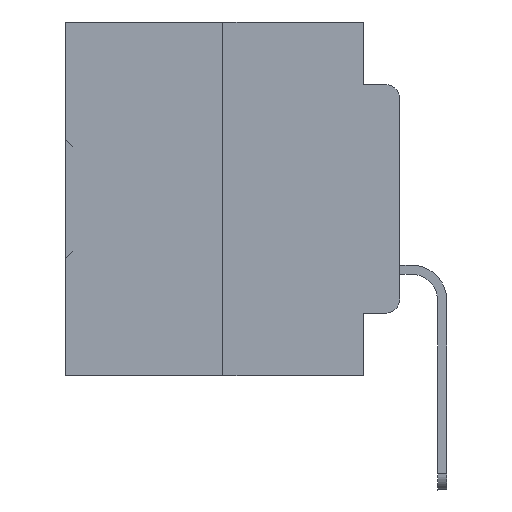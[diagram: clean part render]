
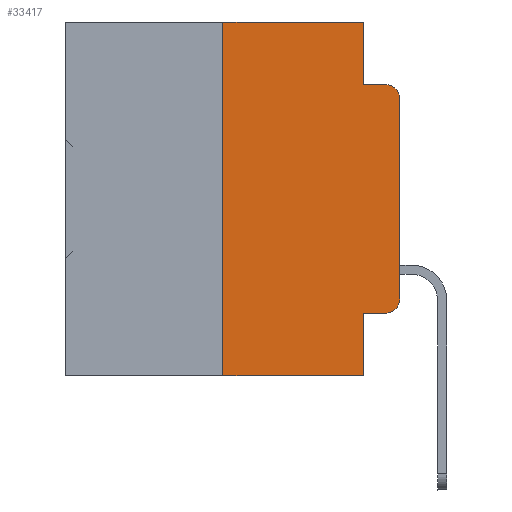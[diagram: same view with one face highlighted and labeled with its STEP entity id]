
A CAD part, left-side view. The second image highlights one B-rep face of the part: STEP entity #33417.
In plain terms, the highlighted planar face has unit normal (-1, 0, 0).
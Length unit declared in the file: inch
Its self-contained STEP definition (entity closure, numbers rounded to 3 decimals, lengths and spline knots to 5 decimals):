
#557 = EDGE_CURVE ( 'NONE', #13613, #4150, #12148, .T. ) ;
#837 = DIRECTION ( 'NONE',  ( 0., -1., 0. ) ) ;
#1370 = VERTEX_POINT ( 'NONE', #20923 ) ;
#1842 = AXIS2_PLACEMENT_3D ( 'NONE', #28471, #22711, #34434 ) ;
#2029 = CARTESIAN_POINT ( 'NONE',  ( 0., 0.02, -0.0885 ) ) ;
#2044 = FACE_OUTER_BOUND ( 'NONE', #7309, .T. ) ;
#2407 = DIRECTION ( 'NONE',  ( -1., 0., 0. ) ) ;
#2476 = ORIENTED_EDGE ( 'NONE', *, *, #37517, .F. ) ;
#2624 = DIRECTION ( 'NONE',  ( 1., 0., 0. ) ) ;
#3008 = EDGE_CURVE ( 'NONE', #10098, #31076, #10506, .T. ) ;
#3671 = EDGE_CURVE ( 'NONE', #20404, #1370, #37446, .T. ) ;
#4150 = VERTEX_POINT ( 'NONE', #14143 ) ;
#4730 = LINE ( 'NONE', #36672, #31308 ) ;
#4738 = CARTESIAN_POINT ( 'NONE',  ( 0., 0.473, 0. ) ) ;
#4822 = ORIENTED_EDGE ( 'NONE', *, *, #557, .F. ) ;
#4982 = AXIS2_PLACEMENT_3D ( 'NONE', #4738, #2624, #28810 ) ;
#5574 = CARTESIAN_POINT ( 'NONE',  ( 0., 0.051, -0.0885 ) ) ;
#5690 = ORIENTED_EDGE ( 'NONE', *, *, #16403, .F. ) ;
#6623 = LINE ( 'NONE', #18384, #8568 ) ;
#7309 = EDGE_LOOP ( 'NONE', ( #28103, #14606, #2476, #34614, #4822, #5690, #7609, #26396, #16035, #16125 ) ) ;
#7523 = VECTOR ( 'NONE', #33469, 39.37008 ) ;
#7609 = ORIENTED_EDGE ( 'NONE', *, *, #3671, .T. ) ;
#7695 = CARTESIAN_POINT ( 'NONE',  ( 0., 0.25, -0.5 ) ) ;
#8011 = DIRECTION ( 'NONE',  ( 0., 0., 1. ) ) ;
#8186 = CARTESIAN_POINT ( 'NONE',  ( 0., 0.02, -0.4115 ) ) ;
#8386 = VERTEX_POINT ( 'NONE', #29024 ) ;
#8568 = VECTOR ( 'NONE', #837, 39.37008 ) ;
#8943 = CARTESIAN_POINT ( 'NONE',  ( 0., 0., -0.3915 ) ) ;
#9642 = VECTOR ( 'NONE', #28596, 39.37008 ) ;
#10098 = VERTEX_POINT ( 'NONE', #8186 ) ;
#10496 = EDGE_CURVE ( 'NONE', #18296, #1370, #11603, .T. ) ;
#10506 = CIRCLE ( 'NONE', #24674, 0.02 ) ;
#11361 = VERTEX_POINT ( 'NONE', #5574 ) ;
#11523 = DIRECTION ( 'NONE',  ( 0., 0., -1. ) ) ;
#11603 = LINE ( 'NONE', #20277, #32957 ) ;
#12123 = VECTOR ( 'NONE', #11523, 39.37008 ) ;
#12148 = LINE ( 'NONE', #23902, #27666 ) ;
#13613 = VERTEX_POINT ( 'NONE', #27407 ) ;
#14143 = CARTESIAN_POINT ( 'NONE',  ( 0., 0.051, 0. ) ) ;
#14606 = ORIENTED_EDGE ( 'NONE', *, *, #38030, .T. ) ;
#16035 = ORIENTED_EDGE ( 'NONE', *, *, #32227, .T. ) ;
#16125 = ORIENTED_EDGE ( 'NONE', *, *, #3008, .T. ) ;
#16403 = EDGE_CURVE ( 'NONE', #20404, #13613, #16863, .T. ) ;
#16815 = DIRECTION ( 'NONE',  ( 0., 0., -1. ) ) ;
#16863 = LINE ( 'NONE', #34179, #9642 ) ;
#18296 = VERTEX_POINT ( 'NONE', #21407 ) ;
#18384 = CARTESIAN_POINT ( 'NONE',  ( 0., 0.051, -0.0885 ) ) ;
#19117 = EDGE_CURVE ( 'NONE', #4150, #11361, #19825, .T. ) ;
#19825 = LINE ( 'NONE', #37867, #12123 ) ;
#20277 = CARTESIAN_POINT ( 'NONE',  ( 0., 0.051, 0. ) ) ;
#20404 = VERTEX_POINT ( 'NONE', #7695 ) ;
#20923 = CARTESIAN_POINT ( 'NONE',  ( 0., 0.051, -0.5 ) ) ;
#21407 = CARTESIAN_POINT ( 'NONE',  ( 0., 0.051, -0.4115 ) ) ;
#22597 = VERTEX_POINT ( 'NONE', #2029 ) ;
#22711 = DIRECTION ( 'NONE',  ( -1., 0., 0. ) ) ;
#23040 = PLANE ( 'NONE',  #4982 ) ;
#23902 = CARTESIAN_POINT ( 'NONE',  ( 0., 0.473, 0. ) ) ;
#24674 = AXIS2_PLACEMENT_3D ( 'NONE', #28782, #2407, #34359 ) ;
#25883 = LINE ( 'NONE', #34704, #31344 ) ;
#26396 = ORIENTED_EDGE ( 'NONE', *, *, #10496, .F. ) ;
#27407 = CARTESIAN_POINT ( 'NONE',  ( 0., 0.25, 0. ) ) ;
#27666 = VECTOR ( 'NONE', #30231, 39.37008 ) ;
#27905 = CARTESIAN_POINT ( 'NONE',  ( 0., 0.473, -0.5 ) ) ;
#28103 = ORIENTED_EDGE ( 'NONE', *, *, #37206, .T. ) ;
#28471 = CARTESIAN_POINT ( 'NONE',  ( 0., 0.02, -0.1085 ) ) ;
#28596 = DIRECTION ( 'NONE',  ( 0., 0., 1. ) ) ;
#28782 = CARTESIAN_POINT ( 'NONE',  ( 0., 0.02, -0.3915 ) ) ;
#28810 = DIRECTION ( 'NONE',  ( 0., 0., -1. ) ) ;
#29024 = CARTESIAN_POINT ( 'NONE',  ( 0., 0., -0.1085 ) ) ;
#30231 = DIRECTION ( 'NONE',  ( 0., -1., 0. ) ) ;
#31076 = VERTEX_POINT ( 'NONE', #8943 ) ;
#31308 = VECTOR ( 'NONE', #8011, 39.37008 ) ;
#31344 = VECTOR ( 'NONE', #37763, 39.37008 ) ;
#32227 = EDGE_CURVE ( 'NONE', #18296, #10098, #25883, .T. ) ;
#32592 = CIRCLE ( 'NONE', #1842, 0.02 ) ;
#32957 = VECTOR ( 'NONE', #16815, 39.37008 ) ;
#33417 = ADVANCED_FACE ( 'NONE', ( #2044 ), #23040, .F. ) ;
#33469 = DIRECTION ( 'NONE',  ( 0., -1., 0. ) ) ;
#34179 = CARTESIAN_POINT ( 'NONE',  ( 0., 0.25, 0. ) ) ;
#34359 = DIRECTION ( 'NONE',  ( 0., 0., -1. ) ) ;
#34434 = DIRECTION ( 'NONE',  ( 0., 0., -1. ) ) ;
#34614 = ORIENTED_EDGE ( 'NONE', *, *, #19117, .F. ) ;
#34704 = CARTESIAN_POINT ( 'NONE',  ( 0., 0.051, -0.4115 ) ) ;
#36672 = CARTESIAN_POINT ( 'NONE',  ( 0., 0., 0. ) ) ;
#37206 = EDGE_CURVE ( 'NONE', #31076, #8386, #4730, .T. ) ;
#37446 = LINE ( 'NONE', #27905, #7523 ) ;
#37517 = EDGE_CURVE ( 'NONE', #11361, #22597, #6623, .T. ) ;
#37763 = DIRECTION ( 'NONE',  ( 0., -1., 0. ) ) ;
#37867 = CARTESIAN_POINT ( 'NONE',  ( 0., 0.051, 0. ) ) ;
#38030 = EDGE_CURVE ( 'NONE', #8386, #22597, #32592, .T. ) ;
